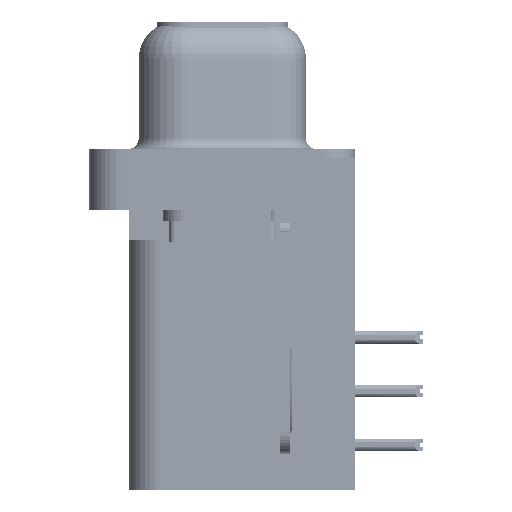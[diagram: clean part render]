
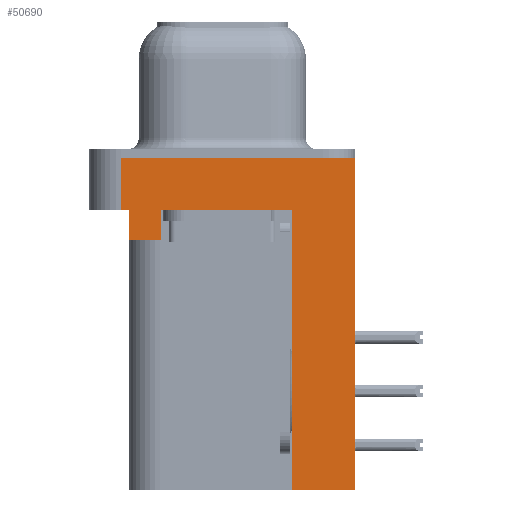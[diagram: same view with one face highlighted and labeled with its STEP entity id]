
A CAD part, left-side view. The second image highlights one B-rep face of the part: STEP entity #50690.
In plain terms, the highlighted planar face has unit normal (-1, 0, 0).
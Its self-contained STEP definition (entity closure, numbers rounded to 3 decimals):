
#253 = ORIENTED_EDGE ( 'NONE', *, *, #35391, .F. ) ;
#1414 = ORIENTED_EDGE ( 'NONE', *, *, #21550, .F. ) ;
#1545 = CARTESIAN_POINT ( 'NONE',  ( -2.91, 2.895, -3.9 ) ) ;
#1567 = CARTESIAN_POINT ( 'NONE',  ( -2.91, 4.425, -3.9 ) ) ;
#2728 = CARTESIAN_POINT ( 'NONE',  ( -2.91, -3.295, -15.7 ) ) ;
#3050 = LINE ( 'NONE', #31568, #11537 ) ;
#3119 = VERTEX_POINT ( 'NONE', #2728 ) ;
#3817 = LINE ( 'NONE', #31019, #13676 ) ;
#5138 = LINE ( 'NONE', #13501, #52806 ) ;
#5157 = VERTEX_POINT ( 'NONE', #46534 ) ;
#5268 = VECTOR ( 'NONE', #52476, 1000. ) ;
#5285 = CARTESIAN_POINT ( 'NONE',  ( -2.91, -6.275, -2.5 ) ) ;
#6058 = CARTESIAN_POINT ( 'NONE',  ( -2.91, -6.275, -2.5 ) ) ;
#6073 = DIRECTION ( 'NONE',  ( 0., 1., 0. ) ) ;
#7209 = VERTEX_POINT ( 'NONE', #34668 ) ;
#7395 = VECTOR ( 'NONE', #23540, 1000. ) ;
#8387 = LINE ( 'NONE', #35377, #52117 ) ;
#8431 = VERTEX_POINT ( 'NONE', #46095 ) ;
#8743 = ORIENTED_EDGE ( 'NONE', *, *, #40848, .F. ) ;
#9985 = DIRECTION ( 'NONE',  ( 0., 0., 1. ) ) ;
#10477 = ORIENTED_EDGE ( 'NONE', *, *, #53544, .T. ) ;
#11537 = VECTOR ( 'NONE', #52723, 1000. ) ;
#13501 = CARTESIAN_POINT ( 'NONE',  ( -2.91, -6.275, 0. ) ) ;
#13676 = VECTOR ( 'NONE', #6073, 1000. ) ;
#13713 = PLANE ( 'NONE',  #20461 ) ;
#16021 = ORIENTED_EDGE ( 'NONE', *, *, #37676, .F. ) ;
#16445 = LINE ( 'NONE', #27110, #5268 ) ;
#16690 = VERTEX_POINT ( 'NONE', #37242 ) ;
#19649 = VECTOR ( 'NONE', #48480, 1000. ) ;
#20141 = VECTOR ( 'NONE', #35881, 1000. ) ;
#20461 = AXIS2_PLACEMENT_3D ( 'NONE', #5285, #47670, #22274 ) ;
#21550 = EDGE_CURVE ( 'NONE', #35389, #7209, #5138, .T. ) ;
#22274 = DIRECTION ( 'NONE',  ( 0., 0., 1. ) ) ;
#23540 = DIRECTION ( 'NONE',  ( 0., 0., 1. ) ) ;
#24922 = VECTOR ( 'NONE', #25203, 1000. ) ;
#25203 = DIRECTION ( 'NONE',  ( 0., 1., 0. ) ) ;
#26040 = CARTESIAN_POINT ( 'NONE',  ( -2.91, -3.295, -2.5 ) ) ;
#26416 = EDGE_LOOP ( 'NONE', ( #1414, #16021, #38729, #31527, #8743, #32804, #10477, #41341, #253, #42564 ) ) ;
#27110 = CARTESIAN_POINT ( 'NONE',  ( -2.91, -6.275, -2.5 ) ) ;
#27777 = VERTEX_POINT ( 'NONE', #35475 ) ;
#29922 = LINE ( 'NONE', #44702, #7395 ) ;
#30856 = LINE ( 'NONE', #6058, #19649 ) ;
#31019 = CARTESIAN_POINT ( 'NONE',  ( -2.91, 4.425, -3.9 ) ) ;
#31527 = ORIENTED_EDGE ( 'NONE', *, *, #36460, .F. ) ;
#31568 = CARTESIAN_POINT ( 'NONE',  ( -2.91, -3.295, -15.7 ) ) ;
#32251 = VERTEX_POINT ( 'NONE', #54508 ) ;
#32804 = ORIENTED_EDGE ( 'NONE', *, *, #47753, .T. ) ;
#33339 = LINE ( 'NONE', #1545, #54583 ) ;
#33450 = CARTESIAN_POINT ( 'NONE',  ( -2.91, -3.295, -15.7 ) ) ;
#34668 = CARTESIAN_POINT ( 'NONE',  ( -2.91, -6.275, 0. ) ) ;
#35053 = EDGE_CURVE ( 'NONE', #5157, #7209, #8387, .T. ) ;
#35166 = DIRECTION ( 'NONE',  ( 0., 0., 1. ) ) ;
#35377 = CARTESIAN_POINT ( 'NONE',  ( -2.91, -6.275, -2.5 ) ) ;
#35389 = VERTEX_POINT ( 'NONE', #42071 ) ;
#35391 = EDGE_CURVE ( 'NONE', #5157, #3119, #36172, .T. ) ;
#35475 = CARTESIAN_POINT ( 'NONE',  ( -2.91, 4.425, -2.5 ) ) ;
#35719 = EDGE_CURVE ( 'NONE', #3119, #44991, #3050, .T. ) ;
#35881 = DIRECTION ( 'NONE',  ( 0., 0., 1. ) ) ;
#36172 = LINE ( 'NONE', #33450, #24922 ) ;
#36460 = EDGE_CURVE ( 'NONE', #45728, #27777, #53899, .T. ) ;
#37242 = CARTESIAN_POINT ( 'NONE',  ( -2.91, 2.895, -3.9 ) ) ;
#37676 = EDGE_CURVE ( 'NONE', #32251, #35389, #29922, .T. ) ;
#38729 = ORIENTED_EDGE ( 'NONE', *, *, #39707, .T. ) ;
#39707 = EDGE_CURVE ( 'NONE', #32251, #27777, #16445, .T. ) ;
#40848 = EDGE_CURVE ( 'NONE', #16690, #45728, #3817, .T. ) ;
#41341 = ORIENTED_EDGE ( 'NONE', *, *, #35719, .F. ) ;
#42071 = CARTESIAN_POINT ( 'NONE',  ( -2.91, 4.775, 0. ) ) ;
#42546 = FACE_OUTER_BOUND ( 'NONE', #26416, .T. ) ;
#42564 = ORIENTED_EDGE ( 'NONE', *, *, #35053, .T. ) ;
#43239 = DIRECTION ( 'NONE',  ( 0., -1., 0. ) ) ;
#44702 = CARTESIAN_POINT ( 'NONE',  ( -2.91, 4.775, -2.5 ) ) ;
#44991 = VERTEX_POINT ( 'NONE', #26040 ) ;
#45728 = VERTEX_POINT ( 'NONE', #1567 ) ;
#46095 = CARTESIAN_POINT ( 'NONE',  ( -2.91, 2.895, -2.5 ) ) ;
#46534 = CARTESIAN_POINT ( 'NONE',  ( -2.91, -6.275, -15.7 ) ) ;
#47670 = DIRECTION ( 'NONE',  ( -1., 0., 0. ) ) ;
#47753 = EDGE_CURVE ( 'NONE', #16690, #8431, #33339, .T. ) ;
#48480 = DIRECTION ( 'NONE',  ( 0., -1., 0. ) ) ;
#48532 = CARTESIAN_POINT ( 'NONE',  ( -2.91, 4.425, -3.9 ) ) ;
#50690 = ADVANCED_FACE ( 'NONE', ( #42546 ), #13713, .T. ) ;
#52117 = VECTOR ( 'NONE', #9985, 1000. ) ;
#52476 = DIRECTION ( 'NONE',  ( 0., -1., 0. ) ) ;
#52723 = DIRECTION ( 'NONE',  ( 0., 0., 1. ) ) ;
#52806 = VECTOR ( 'NONE', #43239, 1000. ) ;
#53544 = EDGE_CURVE ( 'NONE', #8431, #44991, #30856, .T. ) ;
#53899 = LINE ( 'NONE', #48532, #20141 ) ;
#54508 = CARTESIAN_POINT ( 'NONE',  ( -2.91, 4.775, -2.5 ) ) ;
#54583 = VECTOR ( 'NONE', #35166, 1000. ) ;
